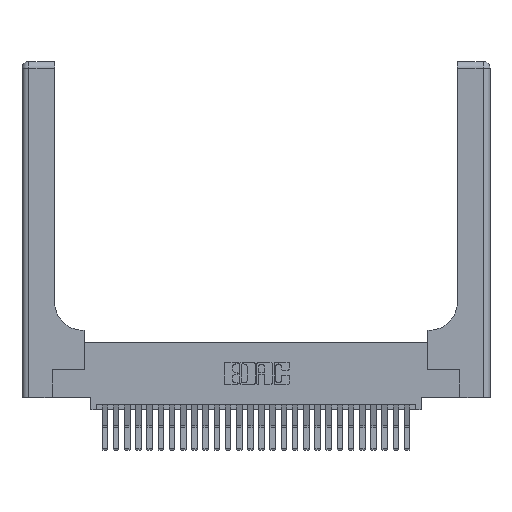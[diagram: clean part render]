
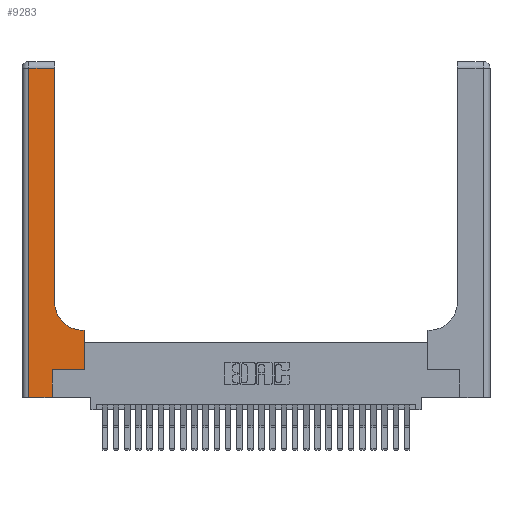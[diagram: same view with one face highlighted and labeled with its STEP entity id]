
A CAD part, top view. The second image highlights one B-rep face of the part: STEP entity #9283.
In plain terms, the highlighted planar face has unit normal (0, 0, 1).
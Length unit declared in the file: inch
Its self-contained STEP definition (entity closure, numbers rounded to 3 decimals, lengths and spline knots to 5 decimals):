
#379 = CARTESIAN_POINT ( 'NONE',  ( 0.5585, 0.25, 0.37 ) ) ;
#558 = CARTESIAN_POINT ( 'NONE',  ( 0.2915, 2.94, 0.37 ) ) ;
#811 = ORIENTED_EDGE ( 'NONE', *, *, #10895, .T. ) ;
#893 = CARTESIAN_POINT ( 'NONE',  ( 0., 0., 0.37 ) ) ;
#1042 = CARTESIAN_POINT ( 'NONE',  ( 0.5415, 0.85, 0.37 ) ) ;
#1684 = LINE ( 'NONE', #24650, #16594 ) ;
#2322 = VERTEX_POINT ( 'NONE', #558 ) ;
#2609 = DIRECTION ( 'NONE',  ( 0., 1., 0. ) ) ;
#2949 = CARTESIAN_POINT ( 'NONE',  ( 0.2915, 0.85, 0.37 ) ) ;
#2993 = ORIENTED_EDGE ( 'NONE', *, *, #10275, .T. ) ;
#3857 = VECTOR ( 'NONE', #22502, 39.37008 ) ;
#3985 = LINE ( 'NONE', #13629, #11077 ) ;
#4559 = EDGE_CURVE ( 'NONE', #10245, #24225, #1684, .T. ) ;
#4646 = EDGE_CURVE ( 'NONE', #22728, #20441, #17953, .T. ) ;
#5025 = CARTESIAN_POINT ( 'NONE',  ( 0.269, 0., 0.37 ) ) ;
#5628 = DIRECTION ( 'NONE',  ( 0., 0., -1. ) ) ;
#5659 = CARTESIAN_POINT ( 'NONE',  ( 0.06, 2.94, 0.37 ) ) ;
#5707 = ORIENTED_EDGE ( 'NONE', *, *, #26521, .T. ) ;
#6824 = CARTESIAN_POINT ( 'NONE',  ( 0.269, 0.25, 0.37 ) ) ;
#7131 = CARTESIAN_POINT ( 'NONE',  ( 0.5415, 0.6, 0.37 ) ) ;
#8355 = CARTESIAN_POINT ( 'NONE',  ( 0., 3., 0.37 ) ) ;
#9283 = ADVANCED_FACE ( 'NONE', ( #17448 ), #26045, .F. ) ;
#9605 = ORIENTED_EDGE ( 'NONE', *, *, #24363, .T. ) ;
#9678 = VERTEX_POINT ( 'NONE', #2949 ) ;
#9751 = VERTEX_POINT ( 'NONE', #5659 ) ;
#9876 = CARTESIAN_POINT ( 'NONE',  ( 0.5585, 0.6, 0.37 ) ) ;
#9907 = LINE ( 'NONE', #15482, #3857 ) ;
#10245 = VERTEX_POINT ( 'NONE', #9876 ) ;
#10275 = EDGE_CURVE ( 'NONE', #25853, #22728, #25185, .T. ) ;
#10349 = DIRECTION ( 'NONE',  ( 0., 0., -1. ) ) ;
#10895 = EDGE_CURVE ( 'NONE', #2322, #9751, #20878, .T. ) ;
#11077 = VECTOR ( 'NONE', #2609, 39.37008 ) ;
#11625 = ORIENTED_EDGE ( 'NONE', *, *, #29002, .T. ) ;
#11659 = CARTESIAN_POINT ( 'NONE',  ( 0., 2.94, 0.37 ) ) ;
#11702 = VECTOR ( 'NONE', #27166, 39.37008 ) ;
#11799 = EDGE_LOOP ( 'NONE', ( #5707, #811, #9605, #2993, #25510, #29022, #11625, #14376, #12749 ) ) ;
#11976 = EDGE_CURVE ( 'NONE', #24225, #9678, #26422, .T. ) ;
#12495 = DIRECTION ( 'NONE',  ( -1., 0., 0. ) ) ;
#12749 = ORIENTED_EDGE ( 'NONE', *, *, #11976, .T. ) ;
#13629 = CARTESIAN_POINT ( 'NONE',  ( 0.5585, 0.25, 0.37 ) ) ;
#14376 = ORIENTED_EDGE ( 'NONE', *, *, #4559, .T. ) ;
#14936 = EDGE_CURVE ( 'NONE', #20441, #24860, #9907, .T. ) ;
#15482 = CARTESIAN_POINT ( 'NONE',  ( 0.269, 0.25, 0.37 ) ) ;
#15596 = VECTOR ( 'NONE', #18561, 39.37008 ) ;
#16594 = VECTOR ( 'NONE', #20254, 39.37008 ) ;
#17448 = FACE_OUTER_BOUND ( 'NONE', #11799, .T. ) ;
#17518 = CARTESIAN_POINT ( 'NONE',  ( 0.2915, 3., 0.37 ) ) ;
#17743 = CARTESIAN_POINT ( 'NONE',  ( 0.06, 0., 0.37 ) ) ;
#17953 = LINE ( 'NONE', #5025, #21852 ) ;
#18426 = AXIS2_PLACEMENT_3D ( 'NONE', #1042, #5628, #23847 ) ;
#18561 = DIRECTION ( 'NONE',  ( 0., -1., 0. ) ) ;
#18959 = LINE ( 'NONE', #17518, #21090 ) ;
#19150 = VECTOR ( 'NONE', #28384, 39.37008 ) ;
#19794 = DIRECTION ( 'NONE',  ( 0., 1., 0. ) ) ;
#20254 = DIRECTION ( 'NONE',  ( -1., 0., 0. ) ) ;
#20441 = VERTEX_POINT ( 'NONE', #6824 ) ;
#20878 = LINE ( 'NONE', #11659, #11702 ) ;
#21090 = VECTOR ( 'NONE', #19794, 39.37008 ) ;
#21852 = VECTOR ( 'NONE', #23236, 39.37008 ) ;
#22502 = DIRECTION ( 'NONE',  ( 1., 0., 0. ) ) ;
#22728 = VERTEX_POINT ( 'NONE', #24334 ) ;
#23236 = DIRECTION ( 'NONE',  ( 0., 1., 0. ) ) ;
#23847 = DIRECTION ( 'NONE',  ( 1., 0., 0. ) ) ;
#24225 = VERTEX_POINT ( 'NONE', #7131 ) ;
#24334 = CARTESIAN_POINT ( 'NONE',  ( 0.269, 0., 0.37 ) ) ;
#24363 = EDGE_CURVE ( 'NONE', #9751, #25853, #28318, .T. ) ;
#24650 = CARTESIAN_POINT ( 'NONE',  ( 0.2915, 0.6, 0.37 ) ) ;
#24860 = VERTEX_POINT ( 'NONE', #379 ) ;
#25185 = LINE ( 'NONE', #893, #19150 ) ;
#25510 = ORIENTED_EDGE ( 'NONE', *, *, #4646, .T. ) ;
#25853 = VERTEX_POINT ( 'NONE', #17743 ) ;
#26045 = PLANE ( 'NONE',  #26845 ) ;
#26422 = CIRCLE ( 'NONE', #18426, 0.25 ) ;
#26521 = EDGE_CURVE ( 'NONE', #9678, #2322, #18959, .T. ) ;
#26845 = AXIS2_PLACEMENT_3D ( 'NONE', #8355, #10349, #12495 ) ;
#27166 = DIRECTION ( 'NONE',  ( -1., 0., 0. ) ) ;
#27660 = CARTESIAN_POINT ( 'NONE',  ( 0.06, 3., 0.37 ) ) ;
#28318 = LINE ( 'NONE', #27660, #15596 ) ;
#28384 = DIRECTION ( 'NONE',  ( 1., 0., 0. ) ) ;
#29002 = EDGE_CURVE ( 'NONE', #24860, #10245, #3985, .T. ) ;
#29022 = ORIENTED_EDGE ( 'NONE', *, *, #14936, .T. ) ;
